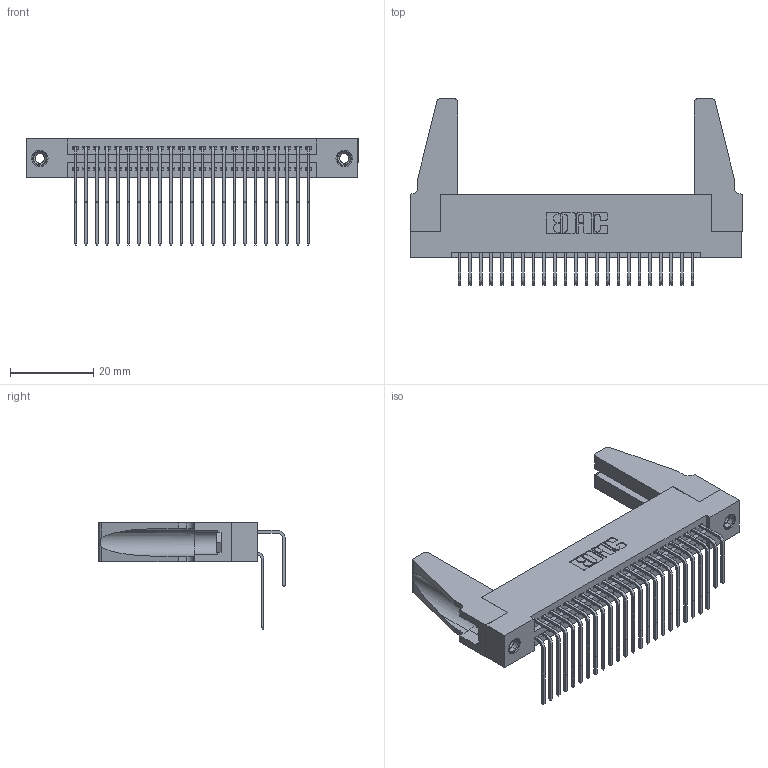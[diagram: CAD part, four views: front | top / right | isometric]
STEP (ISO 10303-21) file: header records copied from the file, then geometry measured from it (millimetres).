
FILE_DESCRIPTION (( 'STEP AP203' ), '1' );
FILE_NAME ('395-046-558-288.STEP', '2019-10-19T04:39:11', ( '' ), ( '' ), 'SwSTEP 2.0', 'SolidWorks 2016', '' );
FILE_SCHEMA (( 'CONFIG_CONTROL_DESIGN' ));
Length unit declared in the file: inch
Products named in the file (6): 345-250-001_345-250-001-102; 345-220-078_345-220-088; 395-046-558-288; 345 Part_Flush Mounting Lugs - 0.156 Dia-TH; 345-292-001_558 559 Tail - 1; 345-292-001_558 Tail - 2
Assembly tree (51 placements, depth 2):
  395-046-558-288
    345 Part_Flush Mounting Lugs - 0.156 Dia-TH
    345-292-001_558 559 Tail - 1  x23
    345-292-001_558 Tail - 2  x23
    345-250-001_345-250-001-102  x2
    345-220-078_345-220-088  x2
Bounding box: 79.65 x 44.69 x 25.53 mm (x, y, z)
Volume: 11079.2 mm3; surface area: 15571.1 mm2
Topology: 51 solids, 51 shells, 2642 faces, 7785 edges, 5118 vertices
Faces by surface type: plane 1762, cylinder 864, cone 12, torus 4
Entity records: 24404 total; most frequent: CARTESIAN_POINT 4149, ORIENTED_EDGE 3992, DIRECTION 3660, EDGE_CURVE 1996, VECTOR 1690, LINE 1690, VERTEX_POINT 1322, AXIS2_PLACEMENT_3D 985
